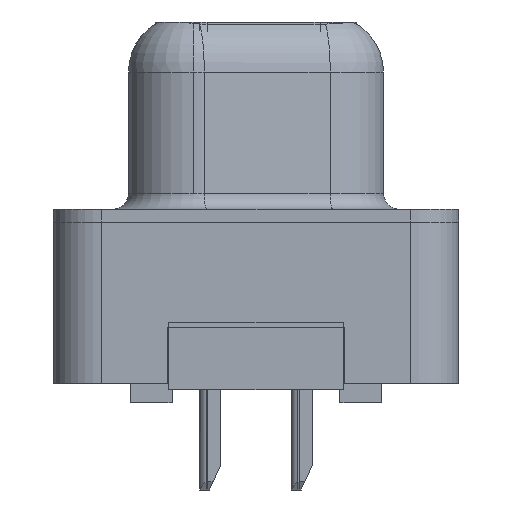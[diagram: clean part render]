
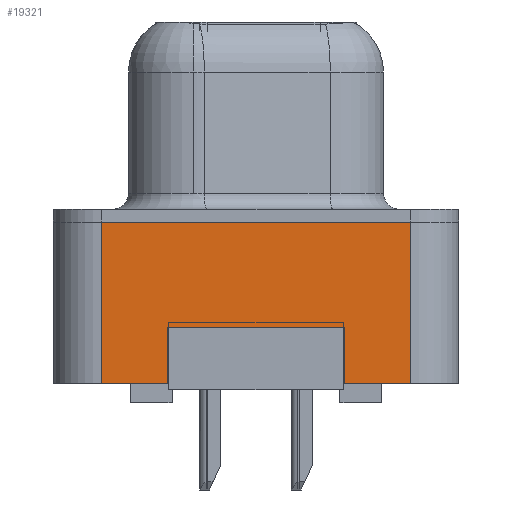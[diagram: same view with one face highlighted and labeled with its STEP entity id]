
A CAD part, left-side view. The second image highlights one B-rep face of the part: STEP entity #19321.
In plain terms, the highlighted planar face has unit normal (-1, 0, 0).
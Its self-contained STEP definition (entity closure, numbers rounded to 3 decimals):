
#252 = CARTESIAN_POINT ( 'NONE',  ( -2.91, -4.775, -5. ) ) ;
#443 = VECTOR ( 'NONE', #21808, 1000. ) ;
#1162 = CARTESIAN_POINT ( 'NONE',  ( -2.91, 4.775, -5. ) ) ;
#1552 = VECTOR ( 'NONE', #1749, 1000. ) ;
#1749 = DIRECTION ( 'NONE',  ( 0., 0., 1. ) ) ;
#1880 = FACE_OUTER_BOUND ( 'NONE', #4630, .T. ) ;
#3286 = ORIENTED_EDGE ( 'NONE', *, *, #6068, .F. ) ;
#3592 = DIRECTION ( 'NONE',  ( -1., 0., 0. ) ) ;
#3810 = CARTESIAN_POINT ( 'NONE',  ( -2.91, -4.775, 0. ) ) ;
#3898 = VECTOR ( 'NONE', #18211, 1000. ) ;
#4328 = ORIENTED_EDGE ( 'NONE', *, *, #5822, .F. ) ;
#4363 = VERTEX_POINT ( 'NONE', #20150 ) ;
#4630 = EDGE_LOOP ( 'NONE', ( #23844, #6267, #9431, #23370, #9794, #8955, #3286, #4328 ) ) ;
#4646 = VECTOR ( 'NONE', #23263, 1000. ) ;
#5069 = DIRECTION ( 'NONE',  ( 0., 0., 1. ) ) ;
#5173 = CARTESIAN_POINT ( 'NONE',  ( -2.91, -4.775, -5. ) ) ;
#5273 = CARTESIAN_POINT ( 'NONE',  ( -2.91, 2.75, -5. ) ) ;
#5398 = LINE ( 'NONE', #5173, #1552 ) ;
#5415 = CARTESIAN_POINT ( 'NONE',  ( -2.91, -4.775, -5. ) ) ;
#5768 = LINE ( 'NONE', #3810, #23025 ) ;
#5822 = EDGE_CURVE ( 'NONE', #14818, #21338, #9935, .T. ) ;
#6018 = DIRECTION ( 'NONE',  ( 0., -1., 0. ) ) ;
#6022 = VERTEX_POINT ( 'NONE', #5273 ) ;
#6068 = EDGE_CURVE ( 'NONE', #21338, #6022, #6856, .T. ) ;
#6267 = ORIENTED_EDGE ( 'NONE', *, *, #15169, .T. ) ;
#6856 = LINE ( 'NONE', #14324, #443 ) ;
#6911 = EDGE_CURVE ( 'NONE', #4363, #21675, #17934, .T. ) ;
#7151 = PLANE ( 'NONE',  #22899 ) ;
#7475 = EDGE_CURVE ( 'NONE', #4363, #6022, #19848, .T. ) ;
#7957 = VERTEX_POINT ( 'NONE', #15757 ) ;
#8622 = DIRECTION ( 'NONE',  ( 0., 0., 1. ) ) ;
#8835 = VERTEX_POINT ( 'NONE', #252 ) ;
#8955 = ORIENTED_EDGE ( 'NONE', *, *, #7475, .T. ) ;
#9431 = ORIENTED_EDGE ( 'NONE', *, *, #11942, .T. ) ;
#9794 = ORIENTED_EDGE ( 'NONE', *, *, #6911, .F. ) ;
#9935 = LINE ( 'NONE', #17418, #4646 ) ;
#11942 = EDGE_CURVE ( 'NONE', #8835, #17166, #5398, .T. ) ;
#12657 = LINE ( 'NONE', #19650, #3898 ) ;
#13813 = EDGE_CURVE ( 'NONE', #21675, #17166, #5768, .T. ) ;
#14324 = CARTESIAN_POINT ( 'NONE',  ( -2.91, 2.75, -3.25 ) ) ;
#14448 = CARTESIAN_POINT ( 'NONE',  ( -2.91, -4.775, -5. ) ) ;
#14818 = VERTEX_POINT ( 'NONE', #21470 ) ;
#15169 = EDGE_CURVE ( 'NONE', #7957, #8835, #17175, .T. ) ;
#15327 = CARTESIAN_POINT ( 'NONE',  ( -2.91, -4.775, -5. ) ) ;
#15443 = DIRECTION ( 'NONE',  ( 0., -1., 0. ) ) ;
#15757 = CARTESIAN_POINT ( 'NONE',  ( -2.91, -2.75, -5. ) ) ;
#16192 = DIRECTION ( 'NONE',  ( 0., -1., 0. ) ) ;
#17166 = VERTEX_POINT ( 'NONE', #19302 ) ;
#17175 = LINE ( 'NONE', #15327, #18036 ) ;
#17418 = CARTESIAN_POINT ( 'NONE',  ( -2.91, 2.75, -3.25 ) ) ;
#17934 = LINE ( 'NONE', #1162, #19353 ) ;
#18036 = VECTOR ( 'NONE', #15443, 1000. ) ;
#18211 = DIRECTION ( 'NONE',  ( 0., 0., -1. ) ) ;
#19302 = CARTESIAN_POINT ( 'NONE',  ( -2.91, -4.775, 0. ) ) ;
#19321 = ADVANCED_FACE ( 'NONE', ( #1880 ), #7151, .T. ) ;
#19353 = VECTOR ( 'NONE', #8622, 1000. ) ;
#19650 = CARTESIAN_POINT ( 'NONE',  ( -2.91, -2.75, -3.25 ) ) ;
#19848 = LINE ( 'NONE', #14448, #22510 ) ;
#20150 = CARTESIAN_POINT ( 'NONE',  ( -2.91, 4.775, -5. ) ) ;
#21106 = CARTESIAN_POINT ( 'NONE',  ( -2.91, 2.75, -3.25 ) ) ;
#21338 = VERTEX_POINT ( 'NONE', #21106 ) ;
#21470 = CARTESIAN_POINT ( 'NONE',  ( -2.91, -2.75, -3.25 ) ) ;
#21675 = VERTEX_POINT ( 'NONE', #23027 ) ;
#21808 = DIRECTION ( 'NONE',  ( 0., 0., -1. ) ) ;
#22510 = VECTOR ( 'NONE', #16192, 1000. ) ;
#22740 = EDGE_CURVE ( 'NONE', #14818, #7957, #12657, .T. ) ;
#22899 = AXIS2_PLACEMENT_3D ( 'NONE', #5415, #3592, #5069 ) ;
#23025 = VECTOR ( 'NONE', #6018, 1000. ) ;
#23027 = CARTESIAN_POINT ( 'NONE',  ( -2.91, 4.775, 0. ) ) ;
#23263 = DIRECTION ( 'NONE',  ( 0., 1., 0. ) ) ;
#23370 = ORIENTED_EDGE ( 'NONE', *, *, #13813, .F. ) ;
#23844 = ORIENTED_EDGE ( 'NONE', *, *, #22740, .T. ) ;
